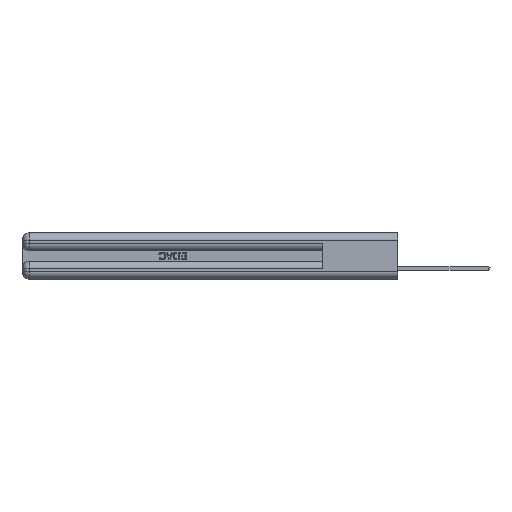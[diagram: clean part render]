
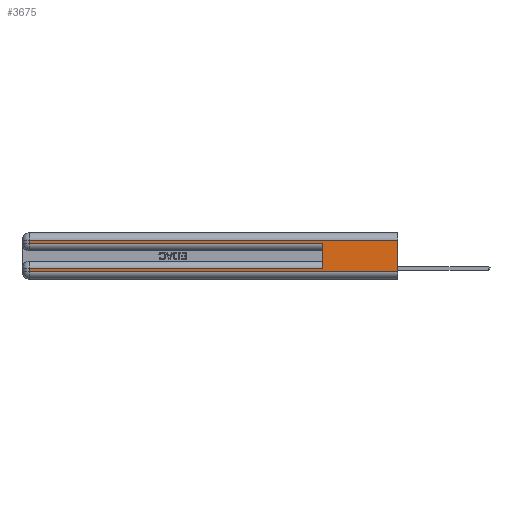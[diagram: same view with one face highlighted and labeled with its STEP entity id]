
A CAD part, left-side view. The second image highlights one B-rep face of the part: STEP entity #3675.
In plain terms, the highlighted planar face has unit normal (-1, 0, 0).
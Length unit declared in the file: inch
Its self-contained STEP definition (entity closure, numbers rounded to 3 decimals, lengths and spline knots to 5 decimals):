
#1208 = CARTESIAN_POINT ( 'NONE',  ( 0., 0., 0.37 ) ) ;
#1970 = DIRECTION ( 'NONE',  ( 0., 0., -1. ) ) ;
#2004 = EDGE_CURVE ( 'NONE', #46533, #21640, #38881, .T. ) ;
#2409 = VERTEX_POINT ( 'NONE', #35522 ) ;
#2671 = VERTEX_POINT ( 'NONE', #25425 ) ;
#3675 = ADVANCED_FACE ( 'NONE', ( #8315 ), #10569, .F. ) ;
#7577 = VECTOR ( 'NONE', #28425, 39.37008 ) ;
#8315 = FACE_OUTER_BOUND ( 'NONE', #34774, .T. ) ;
#9003 = LINE ( 'NONE', #36468, #18236 ) ;
#9618 = ORIENTED_EDGE ( 'NONE', *, *, #38977, .T. ) ;
#9951 = CARTESIAN_POINT ( 'NONE',  ( 0., 2.94, 0.06 ) ) ;
#10569 = PLANE ( 'NONE',  #47323 ) ;
#11223 = EDGE_CURVE ( 'NONE', #2409, #2671, #9003, .T. ) ;
#12169 = DIRECTION ( 'NONE',  ( 0., -1., 0. ) ) ;
#12220 = DIRECTION ( 'NONE',  ( 0., 0., 1. ) ) ;
#14400 = CARTESIAN_POINT ( 'NONE',  ( 0., 0.6, 0.085 ) ) ;
#15106 = CARTESIAN_POINT ( 'NONE',  ( 0., 0.6, 0.285 ) ) ;
#16358 = LINE ( 'NONE', #32233, #26128 ) ;
#16443 = ORIENTED_EDGE ( 'NONE', *, *, #20563, .T. ) ;
#16862 = LINE ( 'NONE', #23717, #7577 ) ;
#17551 = CARTESIAN_POINT ( 'NONE',  ( 0., 2.94, 0.085 ) ) ;
#18063 = ORIENTED_EDGE ( 'NONE', *, *, #2004, .F. ) ;
#18236 = VECTOR ( 'NONE', #29051, 39.37008 ) ;
#20563 = EDGE_CURVE ( 'NONE', #2671, #22499, #42983, .T. ) ;
#21640 = VERTEX_POINT ( 'NONE', #15106 ) ;
#22499 = VERTEX_POINT ( 'NONE', #37521 ) ;
#23432 = EDGE_CURVE ( 'NONE', #46533, #26499, #39942, .T. ) ;
#23717 = CARTESIAN_POINT ( 'NONE',  ( 0., 0., 0.06 ) ) ;
#24751 = DIRECTION ( 'NONE',  ( 0., 1., 0. ) ) ;
#25425 = CARTESIAN_POINT ( 'NONE',  ( 0., 2.94, 0.31 ) ) ;
#26128 = VECTOR ( 'NONE', #12169, 39.37008 ) ;
#26499 = VERTEX_POINT ( 'NONE', #17551 ) ;
#26663 = ORIENTED_EDGE ( 'NONE', *, *, #52924, .T. ) ;
#26938 = VECTOR ( 'NONE', #12220, 39.37008 ) ;
#27805 = DIRECTION ( 'NONE',  ( 0., 0., -1. ) ) ;
#28425 = DIRECTION ( 'NONE',  ( 0., -1., 0. ) ) ;
#28964 = CARTESIAN_POINT ( 'NONE',  ( 0., 0.6, 0.145 ) ) ;
#29051 = DIRECTION ( 'NONE',  ( 0., 1., 0. ) ) ;
#29818 = EDGE_CURVE ( 'NONE', #26499, #52768, #36191, .T. ) ;
#29971 = LINE ( 'NONE', #1208, #33337 ) ;
#31459 = EDGE_CURVE ( 'NONE', #2409, #37879, #29971, .T. ) ;
#32233 = CARTESIAN_POINT ( 'NONE',  ( 0., 0., 0.285 ) ) ;
#32903 = DIRECTION ( 'NONE',  ( 0., 0., -1. ) ) ;
#33337 = VECTOR ( 'NONE', #1970, 39.37008 ) ;
#33869 = ORIENTED_EDGE ( 'NONE', *, *, #11223, .T. ) ;
#34774 = EDGE_LOOP ( 'NONE', ( #46010, #33869, #16443, #9618, #18063, #45443, #50157, #26663 ) ) ;
#35522 = CARTESIAN_POINT ( 'NONE',  ( 0., 0., 0.31 ) ) ;
#36063 = DIRECTION ( 'NONE',  ( 0., 0., -1. ) ) ;
#36191 = LINE ( 'NONE', #46045, #52017 ) ;
#36260 = CARTESIAN_POINT ( 'NONE',  ( 0., 0., 0.37 ) ) ;
#36468 = CARTESIAN_POINT ( 'NONE',  ( 0., 0., 0.31 ) ) ;
#36695 = CARTESIAN_POINT ( 'NONE',  ( 0., 2.94, 0.37 ) ) ;
#37521 = CARTESIAN_POINT ( 'NONE',  ( 0., 2.94, 0.285 ) ) ;
#37879 = VERTEX_POINT ( 'NONE', #41786 ) ;
#38881 = LINE ( 'NONE', #28964, #26938 ) ;
#38977 = EDGE_CURVE ( 'NONE', #22499, #21640, #16358, .T. ) ;
#39942 = LINE ( 'NONE', #46319, #41357 ) ;
#40532 = DIRECTION ( 'NONE',  ( 1., 0., 0. ) ) ;
#41357 = VECTOR ( 'NONE', #24751, 39.37008 ) ;
#41786 = CARTESIAN_POINT ( 'NONE',  ( 0., 0., 0.06 ) ) ;
#42347 = VECTOR ( 'NONE', #27805, 39.37008 ) ;
#42983 = LINE ( 'NONE', #36695, #42347 ) ;
#45443 = ORIENTED_EDGE ( 'NONE', *, *, #23432, .T. ) ;
#46010 = ORIENTED_EDGE ( 'NONE', *, *, #31459, .F. ) ;
#46045 = CARTESIAN_POINT ( 'NONE',  ( 0., 2.94, 0.37 ) ) ;
#46319 = CARTESIAN_POINT ( 'NONE',  ( 0., 0., 0.085 ) ) ;
#46533 = VERTEX_POINT ( 'NONE', #14400 ) ;
#47323 = AXIS2_PLACEMENT_3D ( 'NONE', #36260, #40532, #36063 ) ;
#50157 = ORIENTED_EDGE ( 'NONE', *, *, #29818, .T. ) ;
#52017 = VECTOR ( 'NONE', #32903, 39.37008 ) ;
#52768 = VERTEX_POINT ( 'NONE', #9951 ) ;
#52924 = EDGE_CURVE ( 'NONE', #52768, #37879, #16862, .T. ) ;
